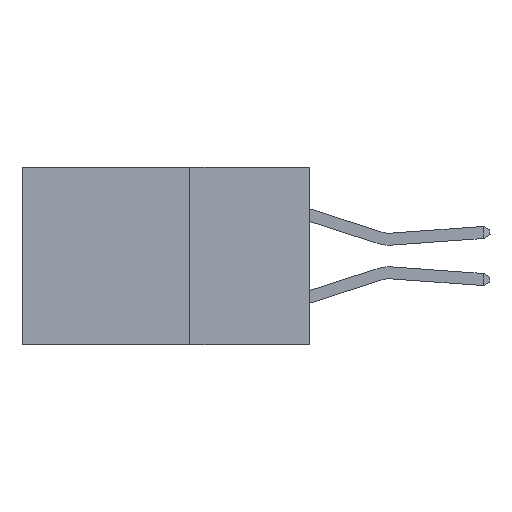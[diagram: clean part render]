
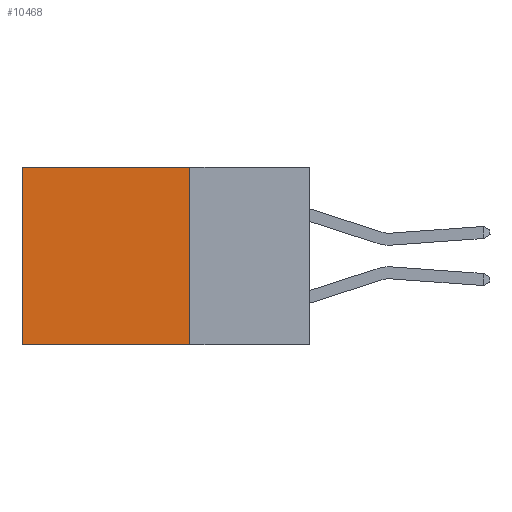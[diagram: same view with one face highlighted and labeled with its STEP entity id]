
A CAD part, left-side view. The second image highlights one B-rep face of the part: STEP entity #10468.
In plain terms, the highlighted planar face has unit normal (-1, 0, 0).
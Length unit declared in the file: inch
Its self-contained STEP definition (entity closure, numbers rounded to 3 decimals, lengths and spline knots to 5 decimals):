
#1085 = DIRECTION ( 'NONE',  ( 0., 1., 0. ) ) ;
#2570 = VERTEX_POINT ( 'NONE', #25706 ) ;
#4412 = CARTESIAN_POINT ( 'NONE',  ( 0.2615, 0.25, 0. ) ) ;
#4855 = VECTOR ( 'NONE', #19787, 39.37008 ) ;
#5861 = CARTESIAN_POINT ( 'NONE',  ( 0.2615, 0.25, -0.37 ) ) ;
#6409 = DIRECTION ( 'NONE',  ( 0., 0., -1. ) ) ;
#6488 = LINE ( 'NONE', #4412, #9414 ) ;
#7733 = VERTEX_POINT ( 'NONE', #5861 ) ;
#8102 = FACE_OUTER_BOUND ( 'NONE', #8152, .T. ) ;
#8152 = EDGE_LOOP ( 'NONE', ( #9045, #20604, #17010, #15887 ) ) ;
#8494 = LINE ( 'NONE', #22212, #11117 ) ;
#9045 = ORIENTED_EDGE ( 'NONE', *, *, #12461, .T. ) ;
#9414 = VECTOR ( 'NONE', #16398, 39.37008 ) ;
#10187 = EDGE_CURVE ( 'NONE', #7733, #16543, #23004, .T. ) ;
#10468 = ADVANCED_FACE ( 'NONE', ( #8102 ), #24025, .F. ) ;
#11117 = VECTOR ( 'NONE', #6409, 39.37008 ) ;
#11228 = AXIS2_PLACEMENT_3D ( 'NONE', #24166, #18137, #20367 ) ;
#12201 = EDGE_CURVE ( 'NONE', #2570, #21808, #6488, .T. ) ;
#12461 = EDGE_CURVE ( 'NONE', #21808, #16543, #15981, .T. ) ;
#13615 = CARTESIAN_POINT ( 'NONE',  ( 0.2615, 0.6, 0. ) ) ;
#15799 = VECTOR ( 'NONE', #1085, 39.37008 ) ;
#15887 = ORIENTED_EDGE ( 'NONE', *, *, #12201, .T. ) ;
#15981 = LINE ( 'NONE', #25654, #4855 ) ;
#16398 = DIRECTION ( 'NONE',  ( 0., 1., 0. ) ) ;
#16543 = VERTEX_POINT ( 'NONE', #17142 ) ;
#17010 = ORIENTED_EDGE ( 'NONE', *, *, #20661, .F. ) ;
#17142 = CARTESIAN_POINT ( 'NONE',  ( 0.2615, 0.6, -0.37 ) ) ;
#18137 = DIRECTION ( 'NONE',  ( 1., 0., 0. ) ) ;
#19787 = DIRECTION ( 'NONE',  ( 0., 0., -1. ) ) ;
#20367 = DIRECTION ( 'NONE',  ( 0., 0., -1. ) ) ;
#20604 = ORIENTED_EDGE ( 'NONE', *, *, #10187, .F. ) ;
#20661 = EDGE_CURVE ( 'NONE', #2570, #7733, #8494, .T. ) ;
#21808 = VERTEX_POINT ( 'NONE', #13615 ) ;
#22212 = CARTESIAN_POINT ( 'NONE',  ( 0.2615, 0.25, -0.37 ) ) ;
#22737 = CARTESIAN_POINT ( 'NONE',  ( 0.2615, 0.25, -0.37 ) ) ;
#23004 = LINE ( 'NONE', #22737, #15799 ) ;
#24025 = PLANE ( 'NONE',  #11228 ) ;
#24166 = CARTESIAN_POINT ( 'NONE',  ( 0.2615, 0.25, -0.37 ) ) ;
#25654 = CARTESIAN_POINT ( 'NONE',  ( 0.2615, 0.6, -0.37 ) ) ;
#25706 = CARTESIAN_POINT ( 'NONE',  ( 0.2615, 0.25, 0. ) ) ;
